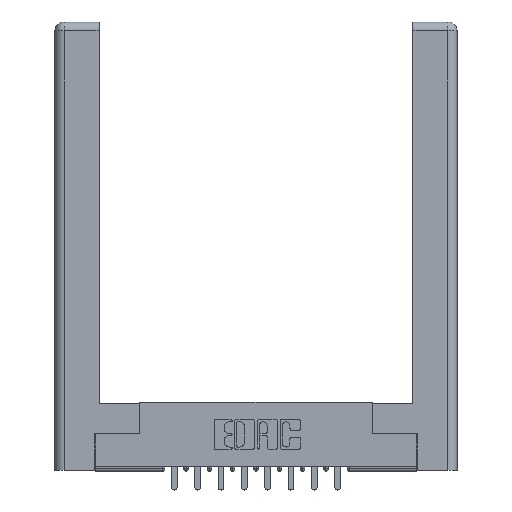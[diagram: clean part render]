
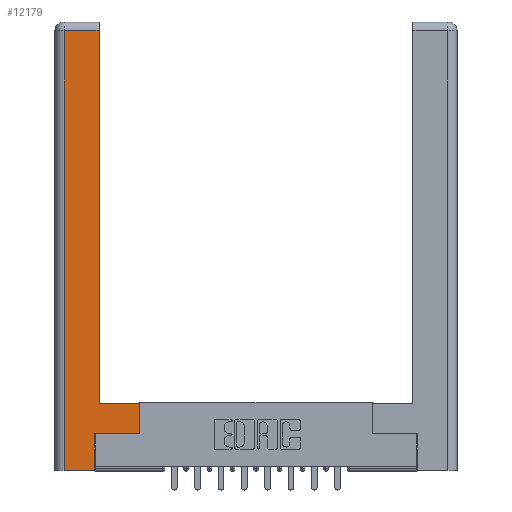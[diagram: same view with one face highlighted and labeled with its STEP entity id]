
A CAD part, top view. The second image highlights one B-rep face of the part: STEP entity #12179.
In plain terms, the highlighted planar face has unit normal (0, 0, 1).
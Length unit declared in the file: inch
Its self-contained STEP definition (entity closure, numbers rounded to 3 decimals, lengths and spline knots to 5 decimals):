
#85 = VECTOR ( 'NONE', #12621, 39.37008 ) ;
#236 = DIRECTION ( 'NONE',  ( 0., 1., 0. ) ) ;
#289 = CARTESIAN_POINT ( 'NONE',  ( 0.565, 0.245, 0. ) ) ;
#324 = AXIS2_PLACEMENT_3D ( 'NONE', #1058, #9065, #2395 ) ;
#442 = EDGE_LOOP ( 'NONE', ( #7163, #11374, #871, #2426, #14157, #9602, #2702, #9729 ) ) ;
#498 = LINE ( 'NONE', #12580, #85 ) ;
#542 = VECTOR ( 'NONE', #2097, 39.37008 ) ;
#596 = CARTESIAN_POINT ( 'NONE',  ( 0.295, 2.94, 0. ) ) ;
#598 = CARTESIAN_POINT ( 'NONE',  ( 0.0615, 2.94, 0. ) ) ;
#871 = ORIENTED_EDGE ( 'NONE', *, *, #12554, .T. ) ;
#1012 = DIRECTION ( 'NONE',  ( 0., 1., 0. ) ) ;
#1058 = CARTESIAN_POINT ( 'NONE',  ( 0., 0., 0. ) ) ;
#1091 = DIRECTION ( 'NONE',  ( -1., 0., 0. ) ) ;
#1252 = VECTOR ( 'NONE', #5216, 39.37008 ) ;
#1589 = CARTESIAN_POINT ( 'NONE',  ( 0.265, 0.245, 0. ) ) ;
#1985 = VERTEX_POINT ( 'NONE', #8210 ) ;
#2097 = DIRECTION ( 'NONE',  ( 0., 1., 0. ) ) ;
#2395 = DIRECTION ( 'NONE',  ( -1., 0., 0. ) ) ;
#2426 = ORIENTED_EDGE ( 'NONE', *, *, #14094, .T. ) ;
#2702 = ORIENTED_EDGE ( 'NONE', *, *, #8205, .T. ) ;
#3934 = LINE ( 'NONE', #10973, #542 ) ;
#4690 = VERTEX_POINT ( 'NONE', #596 ) ;
#5029 = CARTESIAN_POINT ( 'NONE',  ( 0.565, 0.245, 0. ) ) ;
#5041 = CARTESIAN_POINT ( 'NONE',  ( 0.265, 0., 0. ) ) ;
#5135 = EDGE_CURVE ( 'NONE', #11612, #12915, #5258, .T. ) ;
#5216 = DIRECTION ( 'NONE',  ( 1., 0., 0. ) ) ;
#5225 = LINE ( 'NONE', #6873, #8405 ) ;
#5258 = LINE ( 'NONE', #1589, #10284 ) ;
#5279 = VERTEX_POINT ( 'NONE', #10792 ) ;
#6336 = FACE_OUTER_BOUND ( 'NONE', #442, .T. ) ;
#6873 = CARTESIAN_POINT ( 'NONE',  ( 0.565, 0.45, 0. ) ) ;
#6906 = PLANE ( 'NONE',  #324 ) ;
#7136 = VECTOR ( 'NONE', #1091, 39.37008 ) ;
#7163 = ORIENTED_EDGE ( 'NONE', *, *, #9430, .T. ) ;
#7289 = EDGE_CURVE ( 'NONE', #12915, #12451, #10280, .T. ) ;
#7689 = CARTESIAN_POINT ( 'NONE',  ( 0.265, 0.245, 0. ) ) ;
#7799 = VECTOR ( 'NONE', #12502, 39.37008 ) ;
#7934 = CARTESIAN_POINT ( 'NONE',  ( 0.0615, 2.94, 0. ) ) ;
#8205 = EDGE_CURVE ( 'NONE', #12451, #5279, #5225, .T. ) ;
#8210 = CARTESIAN_POINT ( 'NONE',  ( 0.0615, 0., 0. ) ) ;
#8405 = VECTOR ( 'NONE', #1012, 39.37008 ) ;
#9065 = DIRECTION ( 'NONE',  ( 0., 0., -1. ) ) ;
#9289 = VERTEX_POINT ( 'NONE', #11758 ) ;
#9316 = CARTESIAN_POINT ( 'NONE',  ( 0.295, 0.45, 0. ) ) ;
#9430 = EDGE_CURVE ( 'NONE', #9289, #4690, #3934, .T. ) ;
#9602 = ORIENTED_EDGE ( 'NONE', *, *, #7289, .T. ) ;
#9685 = VERTEX_POINT ( 'NONE', #598 ) ;
#9729 = ORIENTED_EDGE ( 'NONE', *, *, #12472, .T. ) ;
#9982 = LINE ( 'NONE', #7934, #7136 ) ;
#10280 = LINE ( 'NONE', #289, #1252 ) ;
#10284 = VECTOR ( 'NONE', #236, 39.37008 ) ;
#10432 = DIRECTION ( 'NONE',  ( -1., 0., 0. ) ) ;
#10792 = CARTESIAN_POINT ( 'NONE',  ( 0.565, 0.45, 0. ) ) ;
#10973 = CARTESIAN_POINT ( 'NONE',  ( 0.295, 3., 0. ) ) ;
#10994 = LINE ( 'NONE', #5041, #7799 ) ;
#11374 = ORIENTED_EDGE ( 'NONE', *, *, #13232, .T. ) ;
#11612 = VERTEX_POINT ( 'NONE', #12686 ) ;
#11758 = CARTESIAN_POINT ( 'NONE',  ( 0.295, 0.45, 0. ) ) ;
#12179 = ADVANCED_FACE ( 'NONE', ( #6336 ), #6906, .F. ) ;
#12451 = VERTEX_POINT ( 'NONE', #5029 ) ;
#12472 = EDGE_CURVE ( 'NONE', #5279, #9289, #13123, .T. ) ;
#12485 = VECTOR ( 'NONE', #10432, 39.37008 ) ;
#12502 = DIRECTION ( 'NONE',  ( 1., 0., 0. ) ) ;
#12554 = EDGE_CURVE ( 'NONE', #9685, #1985, #498, .T. ) ;
#12580 = CARTESIAN_POINT ( 'NONE',  ( 0.0615, 0., 0. ) ) ;
#12621 = DIRECTION ( 'NONE',  ( 0., -1., 0. ) ) ;
#12686 = CARTESIAN_POINT ( 'NONE',  ( 0.265, 0., 0. ) ) ;
#12915 = VERTEX_POINT ( 'NONE', #7689 ) ;
#13123 = LINE ( 'NONE', #9316, #12485 ) ;
#13232 = EDGE_CURVE ( 'NONE', #4690, #9685, #9982, .T. ) ;
#14094 = EDGE_CURVE ( 'NONE', #1985, #11612, #10994, .T. ) ;
#14157 = ORIENTED_EDGE ( 'NONE', *, *, #5135, .T. ) ;
